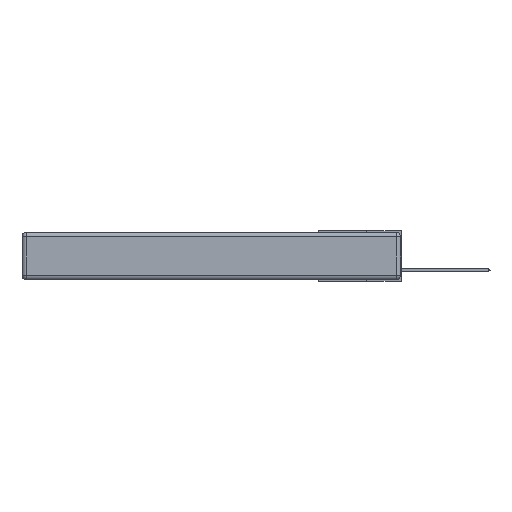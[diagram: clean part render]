
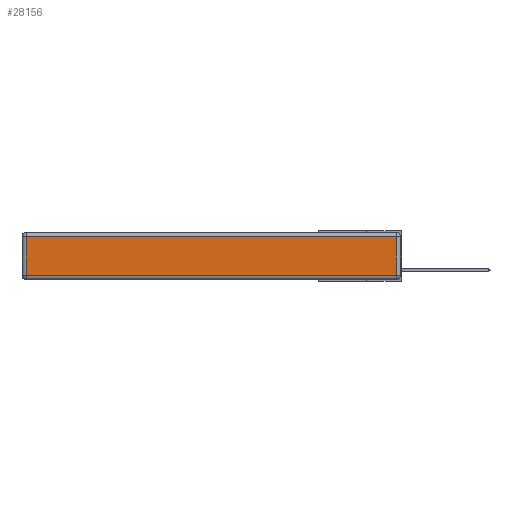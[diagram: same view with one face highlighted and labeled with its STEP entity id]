
A CAD part, left-side view. The second image highlights one B-rep face of the part: STEP entity #28156.
In plain terms, the highlighted planar face has unit normal (-1, 0, 0).
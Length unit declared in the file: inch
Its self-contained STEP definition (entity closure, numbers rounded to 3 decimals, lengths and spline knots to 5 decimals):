
#405 = LINE ( 'NONE', #18589, #20227 ) ;
#518 = ORIENTED_EDGE ( 'NONE', *, *, #11786, .T. ) ;
#1261 = VECTOR ( 'NONE', #10584, 39.37008 ) ;
#3238 = CARTESIAN_POINT ( 'NONE',  ( 0., 2.72, -0.313 ) ) ;
#4768 = VERTEX_POINT ( 'NONE', #27384 ) ;
#6465 = FACE_OUTER_BOUND ( 'NONE', #6692, .T. ) ;
#6692 = EDGE_LOOP ( 'NONE', ( #518, #25822, #18707, #7785 ) ) ;
#6920 = CARTESIAN_POINT ( 'NONE',  ( 0., 0., -0.313 ) ) ;
#7558 = VERTEX_POINT ( 'NONE', #3238 ) ;
#7576 = EDGE_CURVE ( 'NONE', #4768, #27357, #20307, .T. ) ;
#7785 = ORIENTED_EDGE ( 'NONE', *, *, #29815, .T. ) ;
#7899 = CARTESIAN_POINT ( 'NONE',  ( 0., 0.03, -0.343 ) ) ;
#10584 = DIRECTION ( 'NONE',  ( 0., 0., 1. ) ) ;
#10902 = DIRECTION ( 'NONE',  ( 0., 1., 0. ) ) ;
#11786 = EDGE_CURVE ( 'NONE', #7558, #4768, #22707, .T. ) ;
#13020 = EDGE_CURVE ( 'NONE', #27357, #31402, #24884, .T. ) ;
#14160 = DIRECTION ( 'NONE',  ( 0., -1., 0. ) ) ;
#14220 = PLANE ( 'NONE',  #25957 ) ;
#14439 = CARTESIAN_POINT ( 'NONE',  ( 0., 2.72, -0.03 ) ) ;
#14514 = DIRECTION ( 'NONE',  ( -1., 0., 0. ) ) ;
#15878 = CARTESIAN_POINT ( 'NONE',  ( 0., 2.75, -0.03 ) ) ;
#16968 = CARTESIAN_POINT ( 'NONE',  ( 0., 0., -0.343 ) ) ;
#18589 = CARTESIAN_POINT ( 'NONE',  ( 0., 2.72, -0.343 ) ) ;
#18707 = ORIENTED_EDGE ( 'NONE', *, *, #13020, .T. ) ;
#20227 = VECTOR ( 'NONE', #23363, 39.37008 ) ;
#20307 = LINE ( 'NONE', #7899, #1261 ) ;
#22707 = LINE ( 'NONE', #6920, #28392 ) ;
#23363 = DIRECTION ( 'NONE',  ( 0., 0., -1. ) ) ;
#23971 = DIRECTION ( 'NONE',  ( 0., 0., 1. ) ) ;
#24884 = LINE ( 'NONE', #15878, #26388 ) ;
#25822 = ORIENTED_EDGE ( 'NONE', *, *, #7576, .T. ) ;
#25957 = AXIS2_PLACEMENT_3D ( 'NONE', #16968, #14514, #23971 ) ;
#26388 = VECTOR ( 'NONE', #10902, 39.37008 ) ;
#27357 = VERTEX_POINT ( 'NONE', #28017 ) ;
#27384 = CARTESIAN_POINT ( 'NONE',  ( 0., 0.03, -0.313 ) ) ;
#28017 = CARTESIAN_POINT ( 'NONE',  ( 0., 0.03, -0.03 ) ) ;
#28156 = ADVANCED_FACE ( 'NONE', ( #6465 ), #14220, .T. ) ;
#28392 = VECTOR ( 'NONE', #14160, 39.37008 ) ;
#29815 = EDGE_CURVE ( 'NONE', #31402, #7558, #405, .T. ) ;
#31402 = VERTEX_POINT ( 'NONE', #14439 ) ;
